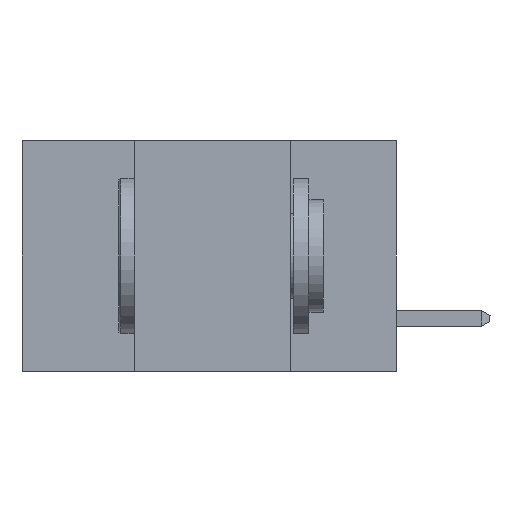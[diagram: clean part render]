
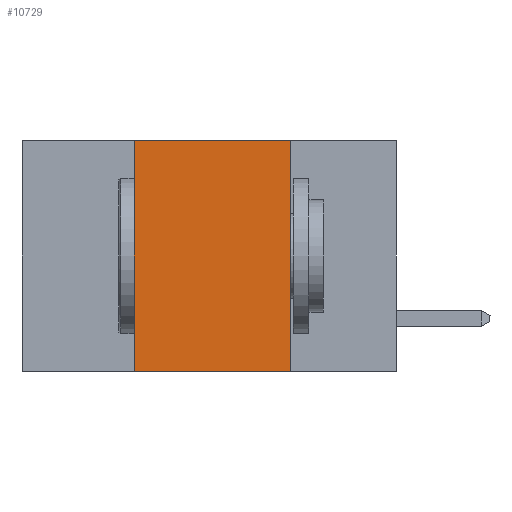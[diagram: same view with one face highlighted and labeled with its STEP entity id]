
A CAD part, left-side view. The second image highlights one B-rep face of the part: STEP entity #10729.
In plain terms, the highlighted planar face has unit normal (-1, 0, 0).
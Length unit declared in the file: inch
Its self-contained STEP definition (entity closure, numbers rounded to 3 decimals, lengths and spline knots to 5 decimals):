
#80 = EDGE_CURVE ( 'NONE', #860, #4617, #12223, .T. ) ;
#357 = VECTOR ( 'NONE', #1774, 39.37008 ) ;
#719 = LINE ( 'NONE', #7029, #357 ) ;
#860 = VERTEX_POINT ( 'NONE', #3587 ) ;
#1581 = CARTESIAN_POINT ( 'NONE',  ( 0., 0.17, 0. ) ) ;
#1774 = DIRECTION ( 'NONE',  ( 0., 0., -1. ) ) ;
#2087 = CARTESIAN_POINT ( 'NONE',  ( 0., 0.42, -0.37 ) ) ;
#3527 = DIRECTION ( 'NONE',  ( 0., -1., 0. ) ) ;
#3587 = CARTESIAN_POINT ( 'NONE',  ( 0., 0.42, -0.37 ) ) ;
#3607 = CARTESIAN_POINT ( 'NONE',  ( 0., 0.6, 0. ) ) ;
#4135 = EDGE_LOOP ( 'NONE', ( #4691, #4938, #5181, #6124 ) ) ;
#4174 = CARTESIAN_POINT ( 'NONE',  ( 0., 0.6, 0. ) ) ;
#4197 = EDGE_CURVE ( 'NONE', #10365, #10990, #8389, .T. ) ;
#4368 = VECTOR ( 'NONE', #10460, 39.37008 ) ;
#4617 = VERTEX_POINT ( 'NONE', #12231 ) ;
#4691 = ORIENTED_EDGE ( 'NONE', *, *, #8430, .F. ) ;
#4938 = ORIENTED_EDGE ( 'NONE', *, *, #4197, .F. ) ;
#5181 = ORIENTED_EDGE ( 'NONE', *, *, #7975, .F. ) ;
#5209 = DIRECTION ( 'NONE',  ( 0., 0., -1. ) ) ;
#5215 = DIRECTION ( 'NONE',  ( 0., 0., 1. ) ) ;
#5887 = LINE ( 'NONE', #2087, #11068 ) ;
#6124 = ORIENTED_EDGE ( 'NONE', *, *, #80, .T. ) ;
#6763 = CARTESIAN_POINT ( 'NONE',  ( 0., 0.42, 0. ) ) ;
#7029 = CARTESIAN_POINT ( 'NONE',  ( 0., 0.17, -0.37 ) ) ;
#7975 = EDGE_CURVE ( 'NONE', #860, #10365, #5887, .T. ) ;
#8389 = LINE ( 'NONE', #3607, #10761 ) ;
#8430 = EDGE_CURVE ( 'NONE', #10990, #4617, #719, .T. ) ;
#9645 = AXIS2_PLACEMENT_3D ( 'NONE', #4174, #11404, #5209 ) ;
#10365 = VERTEX_POINT ( 'NONE', #6763 ) ;
#10398 = PLANE ( 'NONE',  #9645 ) ;
#10460 = DIRECTION ( 'NONE',  ( 0., -1., 0. ) ) ;
#10729 = ADVANCED_FACE ( 'NONE', ( #12513 ), #10398, .F. ) ;
#10761 = VECTOR ( 'NONE', #3527, 39.37008 ) ;
#10990 = VERTEX_POINT ( 'NONE', #1581 ) ;
#11068 = VECTOR ( 'NONE', #5215, 39.37008 ) ;
#11404 = DIRECTION ( 'NONE',  ( 1., 0., 0. ) ) ;
#12223 = LINE ( 'NONE', #12262, #4368 ) ;
#12231 = CARTESIAN_POINT ( 'NONE',  ( 0., 0.17, -0.37 ) ) ;
#12262 = CARTESIAN_POINT ( 'NONE',  ( 0., 0.6, -0.37 ) ) ;
#12513 = FACE_OUTER_BOUND ( 'NONE', #4135, .T. ) ;
